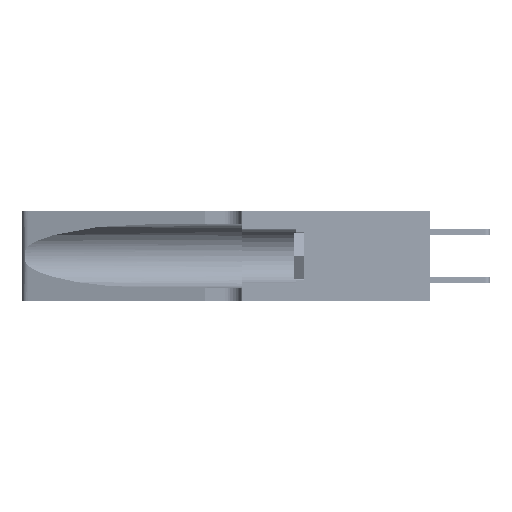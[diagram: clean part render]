
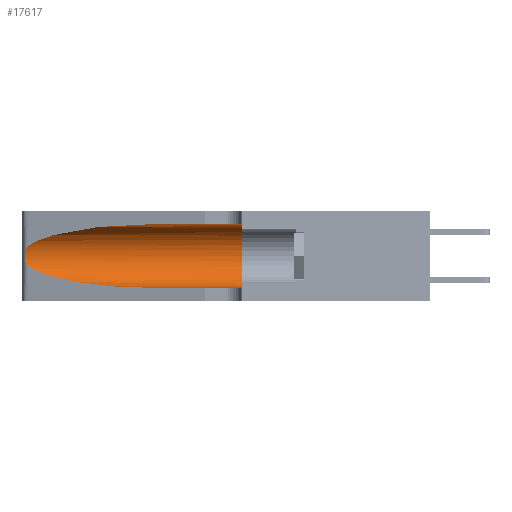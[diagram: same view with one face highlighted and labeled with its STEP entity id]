
A CAD part, left-side view. The second image highlights one B-rep face of the part: STEP entity #17617.
In plain terms, the highlighted cylindrical face has radius 3.308 mm (diameter 6.617 mm), a partial arc.
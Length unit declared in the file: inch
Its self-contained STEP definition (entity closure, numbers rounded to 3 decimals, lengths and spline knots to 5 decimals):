
#1510 = EDGE_CURVE ( 'NONE', #40057, #25671, #44124, .T. ) ;
#1550 = LINE ( 'NONE', #9477, #40289 ) ;
#1816 = LINE ( 'NONE', #48804, #30265 ) ;
#1922 = ORIENTED_EDGE ( 'NONE', *, *, #15612, .T. ) ;
#2813 = CARTESIAN_POINT ( 'NONE',  ( 0.25487, 1.22718, 0.14631 ) ) ;
#3512 = CARTESIAN_POINT ( 'NONE',  ( 0.25639, 1.23184, 0.21858 ) ) ;
#3677 = CARTESIAN_POINT ( 'NONE',  ( 0.25854, 1.2359, 0.20912 ) ) ;
#4556 = FACE_OUTER_BOUND ( 'NONE', #13360, .T. ) ;
#5440 = CARTESIAN_POINT ( 'NONE',  ( 0.1305, 1.61858, 0.185 ) ) ;
#6894 = CARTESIAN_POINT ( 'NONE',  ( 0.25787, 1.23484, 0.2124 ) ) ;
#7077 = CARTESIAN_POINT ( 'NONE',  ( 0.25487, 1.22718, 0.14631 ) ) ;
#8677 = ORIENTED_EDGE ( 'NONE', *, *, #29684, .T. ) ;
#8702 =( BOUNDED_CURVE ( )  B_SPLINE_CURVE ( 3, ( #22391, #21913, #45575, #18180 ),
 .UNSPECIFIED., .F., .T. ) 
 B_SPLINE_CURVE_WITH_KNOTS ( ( 4, 4 ),
 ( 3.44316, 4.71239 ),
 .UNSPECIFIED. ) 
 CURVE ( )  GEOMETRIC_REPRESENTATION_ITEM ( )  RATIONAL_B_SPLINE_CURVE ( ( 1., 0.87, 0.87, 1. ) ) 
 REPRESENTATION_ITEM ( '' )  );
#9477 = CARTESIAN_POINT ( 'NONE',  ( 0.1305, 1.61858, 0.31525 ) ) ;
#12430 =( BOUNDED_CURVE ( )  B_SPLINE_CURVE ( 3, ( #40456, #17294, #44169, #13758 ),
 .UNSPECIFIED., .F., .T. ) 
 B_SPLINE_CURVE_WITH_KNOTS ( ( 4, 4 ),
 ( 1.5708, 2.84003 ),
 .UNSPECIFIED. ) 
 CURVE ( )  GEOMETRIC_REPRESENTATION_ITEM ( )  RATIONAL_B_SPLINE_CURVE ( ( 1., 0.87, 0.87, 1. ) ) 
 REPRESENTATION_ITEM ( '' )  );
#12591 = VERTEX_POINT ( 'NONE', #31033 ) ;
#12910 = AXIS2_PLACEMENT_3D ( 'NONE', #13740, #49724, #22303 ) ;
#13313 = AXIS2_PLACEMENT_3D ( 'NONE', #5440, #13909, #21499 ) ;
#13360 = EDGE_LOOP ( 'NONE', ( #28721, #8677, #16239, #1922, #36238, #27227 ) ) ;
#13740 = CARTESIAN_POINT ( 'NONE',  ( 0.1305, 0.35, 0.185 ) ) ;
#13758 = CARTESIAN_POINT ( 'NONE',  ( 0.25487, 1.22718, 0.22369 ) ) ;
#13909 = DIRECTION ( 'NONE',  ( 0., -1., 0. ) ) ;
#15194 = CARTESIAN_POINT ( 'NONE',  ( 0.26017, 1.23833, 0.17102 ) ) ;
#15612 = EDGE_CURVE ( 'NONE', #12591, #25671, #1816, .T. ) ;
#16239 = ORIENTED_EDGE ( 'NONE', *, *, #41899, .T. ) ;
#16557 = CARTESIAN_POINT ( 'NONE',  ( 0.1305, 0.35, 0.31525 ) ) ;
#16904 = DIRECTION ( 'NONE',  ( 0., -1., 0. ) ) ;
#17294 = CARTESIAN_POINT ( 'NONE',  ( 0.18966, 0.96281, 0.31525 ) ) ;
#17617 = ADVANCED_FACE ( 'NONE', ( #4556 ), #31716, .F. ) ;
#18180 = CARTESIAN_POINT ( 'NONE',  ( 0.1305, 0.72297, 0.05475 ) ) ;
#19065 = CARTESIAN_POINT ( 'NONE',  ( 0.25639, 1.23186, 0.15144 ) ) ;
#20770 = B_SPLINE_CURVE_WITH_KNOTS ( 'NONE', 3,
 ( #22281, #22446, #3512, #6894, #3677, #46131, #49533, #38358, #15194, #49355, #42237, #19065, #30248, #7077 ),
 .UNSPECIFIED., .F., .F.,
 ( 4, 2, 2, 2, 2, 2, 4 ),
 ( 0., 0.00027, 0.00053, 0.00107, 0.0016, 0.00187, 0.00214 ),
 .UNSPECIFIED. ) ;
#21149 = EDGE_CURVE ( 'NONE', #39346, #46038, #12430, .T. ) ;
#21499 = DIRECTION ( 'NONE',  ( 0., 0., -1. ) ) ;
#21913 = CARTESIAN_POINT ( 'NONE',  ( 0.2373, 1.15595, 0.08982 ) ) ;
#22281 = CARTESIAN_POINT ( 'NONE',  ( 0.25487, 1.22718, 0.22369 ) ) ;
#22303 = DIRECTION ( 'NONE',  ( 0., 0., 1. ) ) ;
#22391 = CARTESIAN_POINT ( 'NONE',  ( 0.25487, 1.22718, 0.14631 ) ) ;
#22446 = CARTESIAN_POINT ( 'NONE',  ( 0.25555, 1.22994, 0.2215 ) ) ;
#25671 = VERTEX_POINT ( 'NONE', #25905 ) ;
#25905 = CARTESIAN_POINT ( 'NONE',  ( 0.1305, 0.35, 0.05475 ) ) ;
#27227 = ORIENTED_EDGE ( 'NONE', *, *, #46706, .F. ) ;
#28166 = CARTESIAN_POINT ( 'NONE',  ( 0.1305, 0.72297, 0.31525 ) ) ;
#28721 = ORIENTED_EDGE ( 'NONE', *, *, #21149, .T. ) ;
#29684 = EDGE_CURVE ( 'NONE', #46038, #40313, #20770, .T. ) ;
#30248 = CARTESIAN_POINT ( 'NONE',  ( 0.25555, 1.22993, 0.14849 ) ) ;
#30265 = VECTOR ( 'NONE', #33395, 39.37008 ) ;
#31033 = CARTESIAN_POINT ( 'NONE',  ( 0.1305, 0.72297, 0.05475 ) ) ;
#31716 = CYLINDRICAL_SURFACE ( 'NONE', #13313, 0.13025 ) ;
#33395 = DIRECTION ( 'NONE',  ( 0., -1., 0. ) ) ;
#36238 = ORIENTED_EDGE ( 'NONE', *, *, #1510, .F. ) ;
#38358 = CARTESIAN_POINT ( 'NONE',  ( 0.26075, 1.23896, 0.178 ) ) ;
#39346 = VERTEX_POINT ( 'NONE', #28166 ) ;
#40057 = VERTEX_POINT ( 'NONE', #16557 ) ;
#40289 = VECTOR ( 'NONE', #16904, 39.37008 ) ;
#40313 = VERTEX_POINT ( 'NONE', #2813 ) ;
#40456 = CARTESIAN_POINT ( 'NONE',  ( 0.1305, 0.72297, 0.31525 ) ) ;
#41899 = EDGE_CURVE ( 'NONE', #40313, #12591, #8702, .T. ) ;
#42237 = CARTESIAN_POINT ( 'NONE',  ( 0.25789, 1.23486, 0.15765 ) ) ;
#44124 = CIRCLE ( 'NONE', #12910, 0.13025 ) ;
#44169 = CARTESIAN_POINT ( 'NONE',  ( 0.2373, 1.15595, 0.28018 ) ) ;
#45575 = CARTESIAN_POINT ( 'NONE',  ( 0.18966, 0.96281, 0.05475 ) ) ;
#46038 = VERTEX_POINT ( 'NONE', #48749 ) ;
#46131 = CARTESIAN_POINT ( 'NONE',  ( 0.26018, 1.23835, 0.19895 ) ) ;
#46706 = EDGE_CURVE ( 'NONE', #39346, #40057, #1550, .T. ) ;
#48749 = CARTESIAN_POINT ( 'NONE',  ( 0.25487, 1.22718, 0.22369 ) ) ;
#48804 = CARTESIAN_POINT ( 'NONE',  ( 0.1305, 1.61858, 0.05475 ) ) ;
#49355 = CARTESIAN_POINT ( 'NONE',  ( 0.25856, 1.23593, 0.16098 ) ) ;
#49533 = CARTESIAN_POINT ( 'NONE',  ( 0.26075, 1.23896, 0.19203 ) ) ;
#49724 = DIRECTION ( 'NONE',  ( 0., 1., 0. ) ) ;
